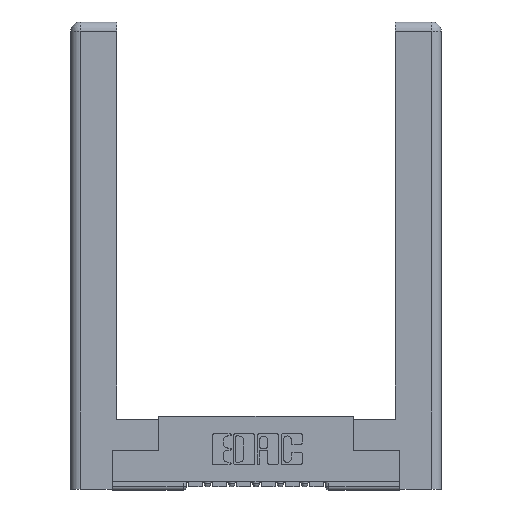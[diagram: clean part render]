
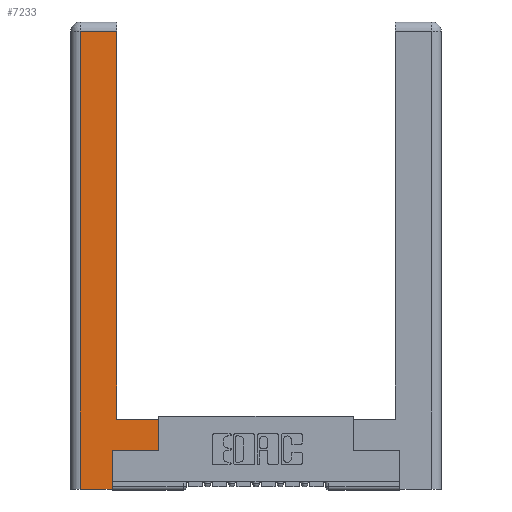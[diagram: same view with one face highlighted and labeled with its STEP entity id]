
A CAD part, top view. The second image highlights one B-rep face of the part: STEP entity #7233.
In plain terms, the highlighted planar face has unit normal (0, 0, 1).
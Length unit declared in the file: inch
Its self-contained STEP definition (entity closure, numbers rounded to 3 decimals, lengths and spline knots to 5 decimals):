
#217 = ORIENTED_EDGE ( 'NONE', *, *, #3977, .T. ) ;
#480 = CARTESIAN_POINT ( 'NONE',  ( 0.565, 0.45, 0. ) ) ;
#500 = ORIENTED_EDGE ( 'NONE', *, *, #10378, .T. ) ;
#527 = VERTEX_POINT ( 'NONE', #1109 ) ;
#546 = DIRECTION ( 'NONE',  ( 0., 0., -1. ) ) ;
#573 = VECTOR ( 'NONE', #12023, 39.37008 ) ;
#761 = VECTOR ( 'NONE', #6465, 39.37008 ) ;
#1109 = CARTESIAN_POINT ( 'NONE',  ( 0.295, 0.45, 0. ) ) ;
#1524 = CARTESIAN_POINT ( 'NONE',  ( 0.295, 3., 0. ) ) ;
#1579 = DIRECTION ( 'NONE',  ( -1., 0., 0. ) ) ;
#1887 = ORIENTED_EDGE ( 'NONE', *, *, #8739, .T. ) ;
#1929 = CARTESIAN_POINT ( 'NONE',  ( 0.565, 0.45, 0. ) ) ;
#1972 = VERTEX_POINT ( 'NONE', #11358 ) ;
#1986 = VECTOR ( 'NONE', #7492, 39.37008 ) ;
#2832 = ORIENTED_EDGE ( 'NONE', *, *, #12162, .T. ) ;
#2997 = CARTESIAN_POINT ( 'NONE',  ( 0.0615, 0., 0. ) ) ;
#3752 = LINE ( 'NONE', #8048, #573 ) ;
#3952 = VERTEX_POINT ( 'NONE', #1929 ) ;
#3977 = EDGE_CURVE ( 'NONE', #5427, #9773, #3752, .T. ) ;
#4009 = DIRECTION ( 'NONE',  ( 0., -1., 0. ) ) ;
#4498 = CARTESIAN_POINT ( 'NONE',  ( 0.295, 2.94, 0. ) ) ;
#5427 = VERTEX_POINT ( 'NONE', #11264 ) ;
#6408 = CARTESIAN_POINT ( 'NONE',  ( 0.565, 0.245, 0. ) ) ;
#6465 = DIRECTION ( 'NONE',  ( 0., 1., 0. ) ) ;
#6888 = EDGE_CURVE ( 'NONE', #3952, #527, #9063, .T. ) ;
#6889 = ORIENTED_EDGE ( 'NONE', *, *, #6888, .T. ) ;
#6940 = LINE ( 'NONE', #480, #761 ) ;
#6968 = VERTEX_POINT ( 'NONE', #9371 ) ;
#7233 = ADVANCED_FACE ( 'NONE', ( #9993 ), #11763, .F. ) ;
#7322 = EDGE_CURVE ( 'NONE', #9207, #12204, #8257, .T. ) ;
#7400 = LINE ( 'NONE', #6408, #1986 ) ;
#7492 = DIRECTION ( 'NONE',  ( 1., 0., 0. ) ) ;
#7583 = LINE ( 'NONE', #7663, #11724 ) ;
#7663 = CARTESIAN_POINT ( 'NONE',  ( 0.265, 0.245, 0. ) ) ;
#7747 = CARTESIAN_POINT ( 'NONE',  ( 0.0615, 2.94, 0. ) ) ;
#7973 = DIRECTION ( 'NONE',  ( -1., 0., 0. ) ) ;
#8048 = CARTESIAN_POINT ( 'NONE',  ( 0.265, 0., 0. ) ) ;
#8234 = EDGE_CURVE ( 'NONE', #1972, #3952, #6940, .T. ) ;
#8257 = LINE ( 'NONE', #8916, #12885 ) ;
#8700 = DIRECTION ( 'NONE',  ( 0., 1., 0. ) ) ;
#8739 = EDGE_CURVE ( 'NONE', #9773, #6968, #7583, .T. ) ;
#8916 = CARTESIAN_POINT ( 'NONE',  ( 0.0615, 2.94, 0. ) ) ;
#8948 = LINE ( 'NONE', #2997, #10671 ) ;
#9063 = LINE ( 'NONE', #10021, #12090 ) ;
#9074 = ORIENTED_EDGE ( 'NONE', *, *, #7322, .T. ) ;
#9207 = VERTEX_POINT ( 'NONE', #4498 ) ;
#9371 = CARTESIAN_POINT ( 'NONE',  ( 0.265, 0.245, 0. ) ) ;
#9773 = VERTEX_POINT ( 'NONE', #10516 ) ;
#9828 = EDGE_LOOP ( 'NONE', ( #2832, #9074, #12261, #217, #1887, #500, #10545, #6889 ) ) ;
#9993 = FACE_OUTER_BOUND ( 'NONE', #9828, .T. ) ;
#10021 = CARTESIAN_POINT ( 'NONE',  ( 0.295, 0.45, 0. ) ) ;
#10378 = EDGE_CURVE ( 'NONE', #6968, #1972, #7400, .T. ) ;
#10516 = CARTESIAN_POINT ( 'NONE',  ( 0.265, 0., 0. ) ) ;
#10545 = ORIENTED_EDGE ( 'NONE', *, *, #8234, .T. ) ;
#10671 = VECTOR ( 'NONE', #4009, 39.37008 ) ;
#10943 = AXIS2_PLACEMENT_3D ( 'NONE', #12745, #546, #1579 ) ;
#11041 = DIRECTION ( 'NONE',  ( -1., 0., 0. ) ) ;
#11264 = CARTESIAN_POINT ( 'NONE',  ( 0.0615, 0., 0. ) ) ;
#11358 = CARTESIAN_POINT ( 'NONE',  ( 0.565, 0.245, 0. ) ) ;
#11579 = DIRECTION ( 'NONE',  ( 0., 1., 0. ) ) ;
#11724 = VECTOR ( 'NONE', #8700, 39.37008 ) ;
#11763 = PLANE ( 'NONE',  #10943 ) ;
#11806 = LINE ( 'NONE', #1524, #12767 ) ;
#11909 = EDGE_CURVE ( 'NONE', #12204, #5427, #8948, .T. ) ;
#12023 = DIRECTION ( 'NONE',  ( 1., 0., 0. ) ) ;
#12090 = VECTOR ( 'NONE', #11041, 39.37008 ) ;
#12162 = EDGE_CURVE ( 'NONE', #527, #9207, #11806, .T. ) ;
#12204 = VERTEX_POINT ( 'NONE', #7747 ) ;
#12261 = ORIENTED_EDGE ( 'NONE', *, *, #11909, .T. ) ;
#12745 = CARTESIAN_POINT ( 'NONE',  ( 0., 0., 0. ) ) ;
#12767 = VECTOR ( 'NONE', #11579, 39.37008 ) ;
#12885 = VECTOR ( 'NONE', #7973, 39.37008 ) ;
